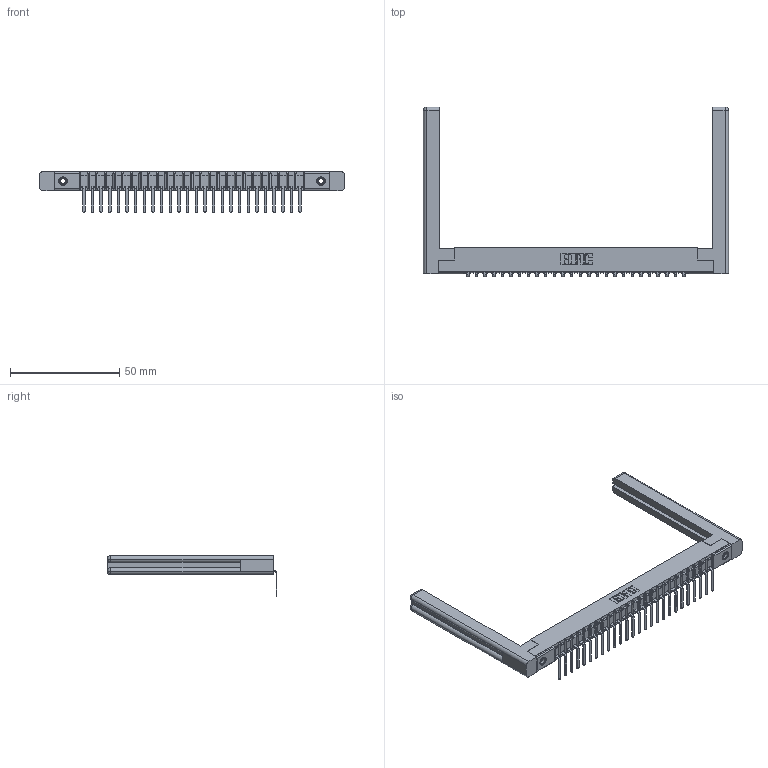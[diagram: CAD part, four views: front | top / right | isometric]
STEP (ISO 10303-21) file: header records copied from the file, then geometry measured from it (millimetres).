
FILE_DESCRIPTION (( 'STEP AP203' ), '1' );
FILE_NAME ('307-026-457-158.STEP', '2020-09-28T04:02:18', ( '' ), ( '' ), 'SwSTEP 2.0', 'SolidWorks 2020', '' );
FILE_SCHEMA (( 'CONFIG_CONTROL_DESIGN' ));
Length unit declared in the file: inch
Products named in the file (5): 307 Part_.156 Dia Mounting Holes; 307-220-058; 345-250-001_345-250-001-102; 307-290-002_557; 307-026-457-158
Assembly tree (31 placements, depth 2):
  307-026-457-158
    307 Part_.156 Dia Mounting Holes
    307-290-002_557  x26
    307-220-058  x2
    345-250-001_345-250-001-102  x2
Bounding box: 139.65 x 77.64 x 18.67 mm (x, y, z)
Volume: 16970 mm3; surface area: 22575.4 mm2
Topology: 31 solids, 31 shells, 2315 faces, 7021 edges, 4594 vertices
Faces by surface type: plane 1376, cylinder 861, sphere 54, torus 12, cone 12
Entity records: 27749 total; most frequent: CARTESIAN_POINT 4687, ORIENTED_EDGE 4616, DIRECTION 4522, EDGE_CURVE 2308, VECTOR 1756, LINE 1756, VERTEX_POINT 1494, AXIS2_PLACEMENT_3D 1383
